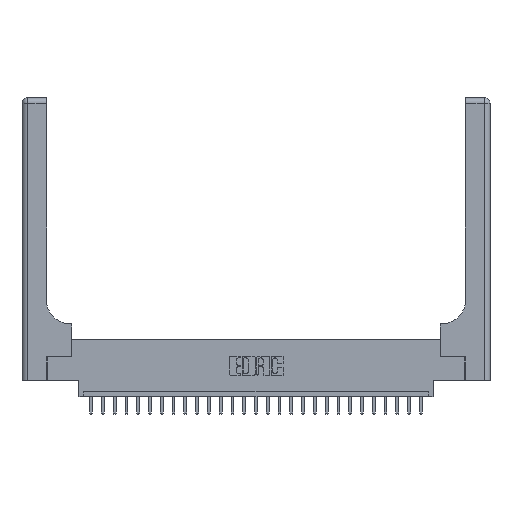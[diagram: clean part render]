
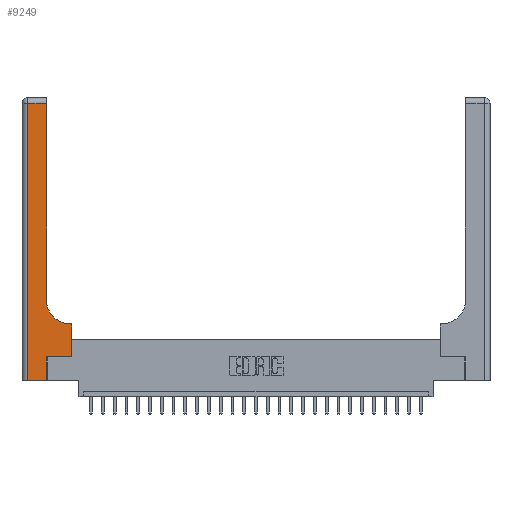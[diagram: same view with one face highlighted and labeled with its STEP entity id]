
A CAD part, top view. The second image highlights one B-rep face of the part: STEP entity #9249.
In plain terms, the highlighted planar face has unit normal (0, 0, 1).
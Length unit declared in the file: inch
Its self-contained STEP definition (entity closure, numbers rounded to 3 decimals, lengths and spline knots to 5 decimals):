
#448 = VECTOR ( 'NONE', #12589, 39.37008 ) ;
#893 = CARTESIAN_POINT ( 'NONE',  ( 0.06, 2.94, 0.37 ) ) ;
#1820 = CARTESIAN_POINT ( 'NONE',  ( 0., 3., 0.37 ) ) ;
#1858 = CARTESIAN_POINT ( 'NONE',  ( 0.06, 3., 0.37 ) ) ;
#2161 = CARTESIAN_POINT ( 'NONE',  ( 0.06, 0., 0.37 ) ) ;
#3002 = VERTEX_POINT ( 'NONE', #15575 ) ;
#3823 = EDGE_CURVE ( 'NONE', #3002, #23850, #4186, .T. ) ;
#3984 = DIRECTION ( 'NONE',  ( 0., 0., -1. ) ) ;
#4186 = LINE ( 'NONE', #17477, #6904 ) ;
#4814 = EDGE_CURVE ( 'NONE', #12324, #21091, #6220, .T. ) ;
#5887 = CARTESIAN_POINT ( 'NONE',  ( 0.26, 3., 0.37 ) ) ;
#5993 = EDGE_CURVE ( 'NONE', #21091, #21122, #7070, .T. ) ;
#6220 = LINE ( 'NONE', #25176, #16064 ) ;
#6904 = VECTOR ( 'NONE', #11555, 39.37008 ) ;
#6934 = DIRECTION ( 'NONE',  ( 1., 0., 0. ) ) ;
#7070 = LINE ( 'NONE', #16440, #448 ) ;
#7278 = VECTOR ( 'NONE', #17663, 39.37008 ) ;
#7529 = ORIENTED_EDGE ( 'NONE', *, *, #4814, .T. ) ;
#8060 = EDGE_CURVE ( 'NONE', #21078, #9294, #22560, .T. ) ;
#8174 = LINE ( 'NONE', #5887, #23109 ) ;
#8493 = EDGE_LOOP ( 'NONE', ( #10868, #11941, #11234, #7529, #15576, #15793, #23294, #15916, #9601 ) ) ;
#8562 = CARTESIAN_POINT ( 'NONE',  ( 0.265, 0., 0.37 ) ) ;
#9249 = ADVANCED_FACE ( 'NONE', ( #15853 ), #13484, .F. ) ;
#9294 = VERTEX_POINT ( 'NONE', #893 ) ;
#9601 = ORIENTED_EDGE ( 'NONE', *, *, #15371, .T. ) ;
#9619 = DIRECTION ( 'NONE',  ( -1., 0., 0. ) ) ;
#10868 = ORIENTED_EDGE ( 'NONE', *, *, #20875, .T. ) ;
#11095 = DIRECTION ( 'NONE',  ( -1., 0., 0. ) ) ;
#11234 = ORIENTED_EDGE ( 'NONE', *, *, #17598, .T. ) ;
#11555 = DIRECTION ( 'NONE',  ( 0., 1., 0. ) ) ;
#11941 = ORIENTED_EDGE ( 'NONE', *, *, #8060, .T. ) ;
#11993 = VECTOR ( 'NONE', #24959, 39.37008 ) ;
#12324 = VERTEX_POINT ( 'NONE', #2161 ) ;
#12402 = CARTESIAN_POINT ( 'NONE',  ( 0.528, 0.6, 0.37 ) ) ;
#12589 = DIRECTION ( 'NONE',  ( 0., 1., 0. ) ) ;
#13484 = PLANE ( 'NONE',  #16516 ) ;
#14350 = LINE ( 'NONE', #1858, #15592 ) ;
#15371 = EDGE_CURVE ( 'NONE', #21253, #19812, #23259, .T. ) ;
#15575 = CARTESIAN_POINT ( 'NONE',  ( 0.528, 0.25, 0.37 ) ) ;
#15576 = ORIENTED_EDGE ( 'NONE', *, *, #5993, .T. ) ;
#15592 = VECTOR ( 'NONE', #23020, 39.37008 ) ;
#15793 = ORIENTED_EDGE ( 'NONE', *, *, #24968, .T. ) ;
#15853 = FACE_OUTER_BOUND ( 'NONE', #8493, .T. ) ;
#15916 = ORIENTED_EDGE ( 'NONE', *, *, #18426, .T. ) ;
#16064 = VECTOR ( 'NONE', #23132, 39.37008 ) ;
#16079 = CARTESIAN_POINT ( 'NONE',  ( 0.26, 0.85, 0.37 ) ) ;
#16188 = DIRECTION ( 'NONE',  ( 0., 1., 0. ) ) ;
#16440 = CARTESIAN_POINT ( 'NONE',  ( 0.265, 0., 0.37 ) ) ;
#16446 = CARTESIAN_POINT ( 'NONE',  ( 0.26, 2.94, 0.37 ) ) ;
#16461 = AXIS2_PLACEMENT_3D ( 'NONE', #23121, #19668, #6934 ) ;
#16516 = AXIS2_PLACEMENT_3D ( 'NONE', #1820, #3984, #9619 ) ;
#16883 = LINE ( 'NONE', #25130, #11993 ) ;
#17477 = CARTESIAN_POINT ( 'NONE',  ( 0.528, 0.25, 0.37 ) ) ;
#17598 = EDGE_CURVE ( 'NONE', #9294, #12324, #14350, .T. ) ;
#17663 = DIRECTION ( 'NONE',  ( -1., 0., 0. ) ) ;
#18426 = EDGE_CURVE ( 'NONE', #23850, #21253, #19485, .T. ) ;
#19485 = LINE ( 'NONE', #24458, #20412 ) ;
#19668 = DIRECTION ( 'NONE',  ( 0., 0., -1. ) ) ;
#19812 = VERTEX_POINT ( 'NONE', #16079 ) ;
#20251 = CARTESIAN_POINT ( 'NONE',  ( 0.265, 0.25, 0.37 ) ) ;
#20412 = VECTOR ( 'NONE', #11095, 39.37008 ) ;
#20875 = EDGE_CURVE ( 'NONE', #19812, #21078, #8174, .T. ) ;
#21078 = VERTEX_POINT ( 'NONE', #16446 ) ;
#21091 = VERTEX_POINT ( 'NONE', #8562 ) ;
#21122 = VERTEX_POINT ( 'NONE', #20251 ) ;
#21253 = VERTEX_POINT ( 'NONE', #22446 ) ;
#22446 = CARTESIAN_POINT ( 'NONE',  ( 0.51, 0.6, 0.37 ) ) ;
#22560 = LINE ( 'NONE', #23413, #7278 ) ;
#23020 = DIRECTION ( 'NONE',  ( 0., -1., 0. ) ) ;
#23109 = VECTOR ( 'NONE', #16188, 39.37008 ) ;
#23121 = CARTESIAN_POINT ( 'NONE',  ( 0.51, 0.85, 0.37 ) ) ;
#23132 = DIRECTION ( 'NONE',  ( 1., 0., 0. ) ) ;
#23259 = CIRCLE ( 'NONE', #16461, 0.25 ) ;
#23294 = ORIENTED_EDGE ( 'NONE', *, *, #3823, .T. ) ;
#23413 = CARTESIAN_POINT ( 'NONE',  ( 0., 2.94, 0.37 ) ) ;
#23850 = VERTEX_POINT ( 'NONE', #12402 ) ;
#24458 = CARTESIAN_POINT ( 'NONE',  ( 0.26, 0.6, 0.37 ) ) ;
#24959 = DIRECTION ( 'NONE',  ( 1., 0., 0. ) ) ;
#24968 = EDGE_CURVE ( 'NONE', #21122, #3002, #16883, .T. ) ;
#25130 = CARTESIAN_POINT ( 'NONE',  ( 0.265, 0.25, 0.37 ) ) ;
#25176 = CARTESIAN_POINT ( 'NONE',  ( 0., 0., 0.37 ) ) ;
